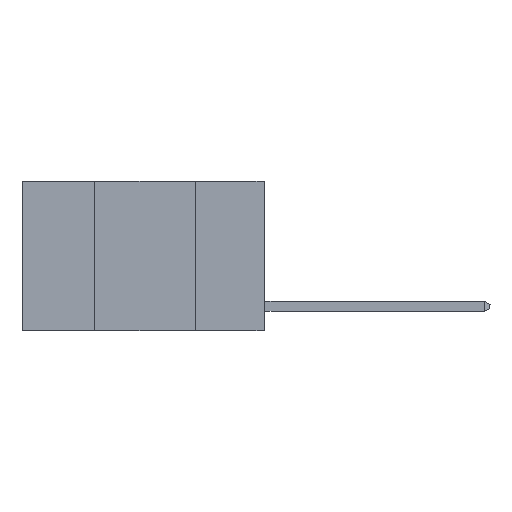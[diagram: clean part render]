
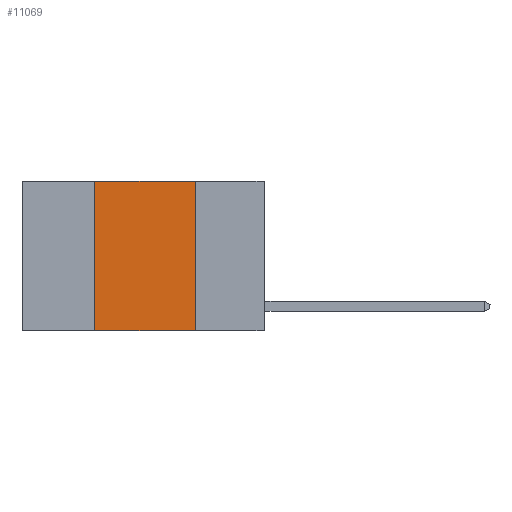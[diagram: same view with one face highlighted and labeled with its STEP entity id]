
A CAD part, left-side view. The second image highlights one B-rep face of the part: STEP entity #11069.
In plain terms, the highlighted planar face has unit normal (-1, 0, 0).
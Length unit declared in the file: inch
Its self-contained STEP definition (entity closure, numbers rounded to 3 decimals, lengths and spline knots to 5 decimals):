
#61 = LINE ( 'NONE', #2180, #6787 ) ;
#212 = VERTEX_POINT ( 'NONE', #711 ) ;
#711 = CARTESIAN_POINT ( 'NONE',  ( 0., 0.17, 0. ) ) ;
#1074 = VERTEX_POINT ( 'NONE', #6313 ) ;
#1355 = VERTEX_POINT ( 'NONE', #7546 ) ;
#1437 = CARTESIAN_POINT ( 'NONE',  ( 0., 0.42, 0. ) ) ;
#1522 = VECTOR ( 'NONE', #6190, 39.37008 ) ;
#1568 = CARTESIAN_POINT ( 'NONE',  ( 0., 0.6, 0. ) ) ;
#1792 = CARTESIAN_POINT ( 'NONE',  ( 0., 0.17, 0. ) ) ;
#1910 = EDGE_CURVE ( 'NONE', #1355, #1074, #61, .T. ) ;
#2042 = ORIENTED_EDGE ( 'NONE', *, *, #1910, .T. ) ;
#2146 = ORIENTED_EDGE ( 'NONE', *, *, #7229, .F. ) ;
#2180 = CARTESIAN_POINT ( 'NONE',  ( 0., 0.6, -0.37 ) ) ;
#2496 = CARTESIAN_POINT ( 'NONE',  ( 0., 0.6, 0. ) ) ;
#2544 = VECTOR ( 'NONE', #4208, 39.37008 ) ;
#2958 = ORIENTED_EDGE ( 'NONE', *, *, #9345, .F. ) ;
#4208 = DIRECTION ( 'NONE',  ( 0., -1., 0. ) ) ;
#4401 = AXIS2_PLACEMENT_3D ( 'NONE', #2496, #11283, #6044 ) ;
#4903 = CARTESIAN_POINT ( 'NONE',  ( 0., 0.42, 0. ) ) ;
#4992 = DIRECTION ( 'NONE',  ( 0., 0., 1. ) ) ;
#5471 = VERTEX_POINT ( 'NONE', #4903 ) ;
#5844 = VECTOR ( 'NONE', #4992, 39.37008 ) ;
#5992 = EDGE_LOOP ( 'NONE', ( #2958, #2146, #11083, #2042 ) ) ;
#6005 = PLANE ( 'NONE',  #4401 ) ;
#6044 = DIRECTION ( 'NONE',  ( 0., 0., -1. ) ) ;
#6121 = LINE ( 'NONE', #1437, #5844 ) ;
#6190 = DIRECTION ( 'NONE',  ( 0., 0., -1. ) ) ;
#6313 = CARTESIAN_POINT ( 'NONE',  ( 0., 0.17, -0.37 ) ) ;
#6592 = FACE_OUTER_BOUND ( 'NONE', #5992, .T. ) ;
#6787 = VECTOR ( 'NONE', #9206, 39.37008 ) ;
#7229 = EDGE_CURVE ( 'NONE', #5471, #212, #9560, .T. ) ;
#7546 = CARTESIAN_POINT ( 'NONE',  ( 0., 0.42, -0.37 ) ) ;
#7786 = EDGE_CURVE ( 'NONE', #1355, #5471, #6121, .T. ) ;
#8512 = LINE ( 'NONE', #1792, #1522 ) ;
#9206 = DIRECTION ( 'NONE',  ( 0., -1., 0. ) ) ;
#9345 = EDGE_CURVE ( 'NONE', #212, #1074, #8512, .T. ) ;
#9560 = LINE ( 'NONE', #1568, #2544 ) ;
#11069 = ADVANCED_FACE ( 'NONE', ( #6592 ), #6005, .F. ) ;
#11083 = ORIENTED_EDGE ( 'NONE', *, *, #7786, .F. ) ;
#11283 = DIRECTION ( 'NONE',  ( 1., 0., 0. ) ) ;
